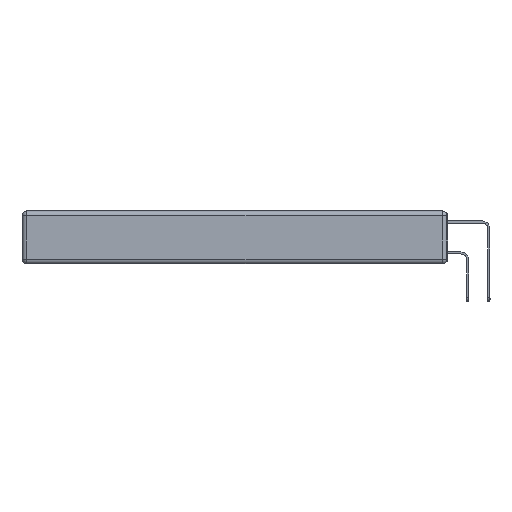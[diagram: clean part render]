
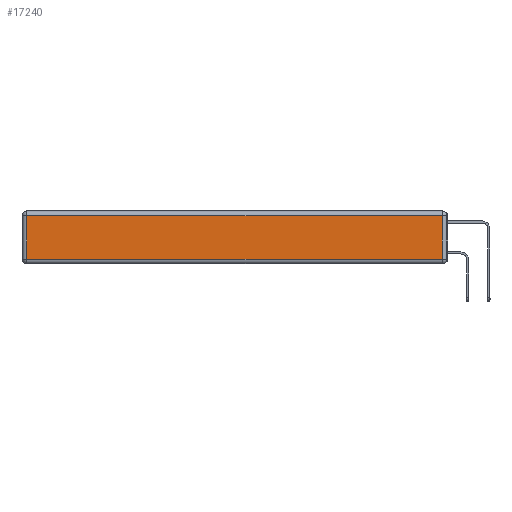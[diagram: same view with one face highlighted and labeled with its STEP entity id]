
A CAD part, left-side view. The second image highlights one B-rep face of the part: STEP entity #17240.
In plain terms, the highlighted planar face has unit normal (-1, 0, 0).
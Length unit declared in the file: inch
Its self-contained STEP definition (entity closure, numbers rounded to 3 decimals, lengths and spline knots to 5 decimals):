
#375 = ORIENTED_EDGE ( 'NONE', *, *, #13362, .T. ) ;
#1651 = PLANE ( 'NONE',  #6759 ) ;
#1955 = VERTEX_POINT ( 'NONE', #15047 ) ;
#2368 = VECTOR ( 'NONE', #16770, 39.37008 ) ;
#3511 = DIRECTION ( 'NONE',  ( 0., 0., 1. ) ) ;
#4399 = DIRECTION ( 'NONE',  ( 0., 0., -1. ) ) ;
#5203 = CARTESIAN_POINT ( 'NONE',  ( 0., 0.03, -0.03 ) ) ;
#6189 = LINE ( 'NONE', #16535, #16549 ) ;
#6759 = AXIS2_PLACEMENT_3D ( 'NONE', #20120, #16465, #3511 ) ;
#7247 = LINE ( 'NONE', #14938, #2368 ) ;
#7369 = DIRECTION ( 'NONE',  ( 0., -1., 0. ) ) ;
#7384 = VERTEX_POINT ( 'NONE', #8669 ) ;
#8363 = CARTESIAN_POINT ( 'NONE',  ( 0., 0.03, -0.343 ) ) ;
#8669 = CARTESIAN_POINT ( 'NONE',  ( 0., 0.03, -0.313 ) ) ;
#8982 = CARTESIAN_POINT ( 'NONE',  ( 0., 2.72, -0.313 ) ) ;
#11522 = ORIENTED_EDGE ( 'NONE', *, *, #23496, .T. ) ;
#13362 = EDGE_CURVE ( 'NONE', #14536, #1955, #7247, .T. ) ;
#13737 = ORIENTED_EDGE ( 'NONE', *, *, #19311, .T. ) ;
#14004 = LINE ( 'NONE', #17375, #21541 ) ;
#14536 = VERTEX_POINT ( 'NONE', #5203 ) ;
#14938 = CARTESIAN_POINT ( 'NONE',  ( 0., 2.75, -0.03 ) ) ;
#15047 = CARTESIAN_POINT ( 'NONE',  ( 0., 2.72, -0.03 ) ) ;
#15883 = VECTOR ( 'NONE', #19430, 39.37008 ) ;
#16465 = DIRECTION ( 'NONE',  ( -1., 0., 0. ) ) ;
#16535 = CARTESIAN_POINT ( 'NONE',  ( 0., 0., -0.313 ) ) ;
#16549 = VECTOR ( 'NONE', #7369, 39.37008 ) ;
#16770 = DIRECTION ( 'NONE',  ( 0., 1., 0. ) ) ;
#17210 = VERTEX_POINT ( 'NONE', #8982 ) ;
#17240 = ADVANCED_FACE ( 'NONE', ( #22495 ), #1651, .T. ) ;
#17375 = CARTESIAN_POINT ( 'NONE',  ( 0., 2.72, -0.343 ) ) ;
#18808 = LINE ( 'NONE', #8363, #15883 ) ;
#18822 = EDGE_CURVE ( 'NONE', #1955, #17210, #14004, .T. ) ;
#18828 = EDGE_LOOP ( 'NONE', ( #13737, #11522, #375, #20052 ) ) ;
#19311 = EDGE_CURVE ( 'NONE', #17210, #7384, #6189, .T. ) ;
#19430 = DIRECTION ( 'NONE',  ( 0., 0., 1. ) ) ;
#20052 = ORIENTED_EDGE ( 'NONE', *, *, #18822, .T. ) ;
#20120 = CARTESIAN_POINT ( 'NONE',  ( 0., 0., -0.343 ) ) ;
#21541 = VECTOR ( 'NONE', #4399, 39.37008 ) ;
#22495 = FACE_OUTER_BOUND ( 'NONE', #18828, .T. ) ;
#23496 = EDGE_CURVE ( 'NONE', #7384, #14536, #18808, .T. ) ;
